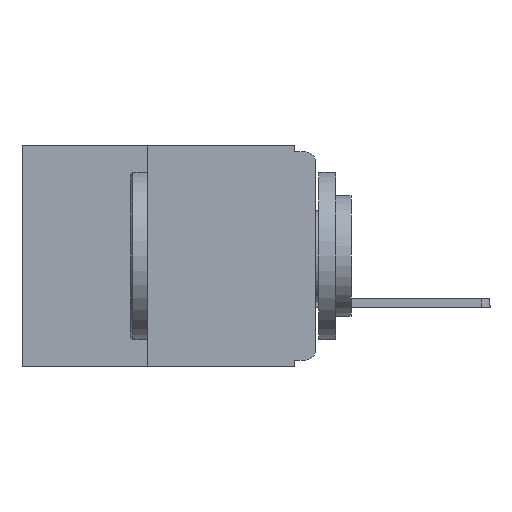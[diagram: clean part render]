
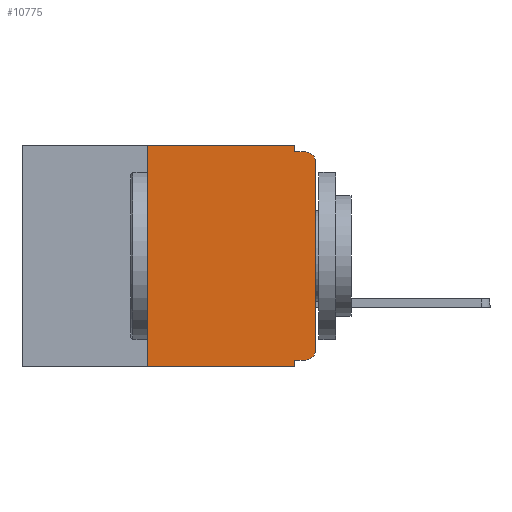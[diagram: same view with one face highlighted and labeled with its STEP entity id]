
A CAD part, left-side view. The second image highlights one B-rep face of the part: STEP entity #10775.
In plain terms, the highlighted planar face has unit normal (-1, 0, 0).
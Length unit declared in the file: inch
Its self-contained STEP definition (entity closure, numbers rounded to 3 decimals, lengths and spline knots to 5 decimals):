
#766 = ORIENTED_EDGE ( 'NONE', *, *, #19208, .F. ) ;
#1764 = DIRECTION ( 'NONE',  ( 0., -1., 0. ) ) ;
#1900 = CARTESIAN_POINT ( 'NONE',  ( 0., 0.015, -0.305 ) ) ;
#2161 = CARTESIAN_POINT ( 'NONE',  ( 0., 0., -0.32 ) ) ;
#3280 = EDGE_LOOP ( 'NONE', ( #29808, #20741, #8644, #12980, #18042, #766, #25653, #30674, #28426, #8640 ) ) ;
#3345 = CARTESIAN_POINT ( 'NONE',  ( 0., 0.25, 0. ) ) ;
#3625 = AXIS2_PLACEMENT_3D ( 'NONE', #1900, #20835, #4644 ) ;
#4491 = LINE ( 'NONE', #29049, #32225 ) ;
#4515 = LINE ( 'NONE', #10232, #24343 ) ;
#4644 = DIRECTION ( 'NONE',  ( 0., 0., -1. ) ) ;
#4915 = DIRECTION ( 'NONE',  ( 0., 1., 0. ) ) ;
#5037 = EDGE_CURVE ( 'NONE', #18623, #21299, #11745, .T. ) ;
#6126 = VECTOR ( 'NONE', #12743, 39.37008 ) ;
#6256 = CARTESIAN_POINT ( 'NONE',  ( 0., 0., -0.305 ) ) ;
#6381 = EDGE_CURVE ( 'NONE', #29842, #32812, #9948, .T. ) ;
#6415 = DIRECTION ( 'NONE',  ( 0., 0., 1. ) ) ;
#6473 = CARTESIAN_POINT ( 'NONE',  ( 0., 0.031, 0. ) ) ;
#6485 = EDGE_CURVE ( 'NONE', #15979, #17301, #20900, .T. ) ;
#7146 = CARTESIAN_POINT ( 'NONE',  ( 0., 0.25, -0.33 ) ) ;
#7497 = DIRECTION ( 'NONE',  ( 0., -1., 0. ) ) ;
#7969 = CARTESIAN_POINT ( 'NONE',  ( 0., 0.015, -0.025 ) ) ;
#8640 = ORIENTED_EDGE ( 'NONE', *, *, #31107, .T. ) ;
#8644 = ORIENTED_EDGE ( 'NONE', *, *, #5037, .F. ) ;
#8775 = CARTESIAN_POINT ( 'NONE',  ( 0., 0., -0.025 ) ) ;
#9948 = LINE ( 'NONE', #2161, #23394 ) ;
#10037 = CARTESIAN_POINT ( 'NONE',  ( 0., 0.031, -0.33 ) ) ;
#10232 = CARTESIAN_POINT ( 'NONE',  ( 0., 0.437, 0. ) ) ;
#10708 = DIRECTION ( 'NONE',  ( 0., 0., -1. ) ) ;
#10775 = ADVANCED_FACE ( 'NONE', ( #24810 ), #29606, .F. ) ;
#11642 = EDGE_CURVE ( 'NONE', #32002, #33208, #32650, .T. ) ;
#11745 = LINE ( 'NONE', #18168, #18114 ) ;
#12477 = CARTESIAN_POINT ( 'NONE',  ( 0., 0.031, -0.32 ) ) ;
#12743 = DIRECTION ( 'NONE',  ( 0., 0., -1. ) ) ;
#12980 = ORIENTED_EDGE ( 'NONE', *, *, #33434, .F. ) ;
#13438 = CARTESIAN_POINT ( 'NONE',  ( 0., 0.437, -0.33 ) ) ;
#13593 = DIRECTION ( 'NONE',  ( 1., 0., 0. ) ) ;
#14656 = LINE ( 'NONE', #20573, #28015 ) ;
#14970 = VERTEX_POINT ( 'NONE', #6473 ) ;
#15979 = VERTEX_POINT ( 'NONE', #7146 ) ;
#16168 = EDGE_CURVE ( 'NONE', #33208, #21299, #20493, .T. ) ;
#16734 = AXIS2_PLACEMENT_3D ( 'NONE', #21576, #13593, #32283 ) ;
#17301 = VERTEX_POINT ( 'NONE', #32049 ) ;
#17327 = CARTESIAN_POINT ( 'NONE',  ( 0., 0., 0. ) ) ;
#17913 = CARTESIAN_POINT ( 'NONE',  ( 0., 0.015, -0.32 ) ) ;
#18042 = ORIENTED_EDGE ( 'NONE', *, *, #32919, .F. ) ;
#18114 = VECTOR ( 'NONE', #1764, 39.37008 ) ;
#18168 = CARTESIAN_POINT ( 'NONE',  ( 0., 0., -0.01 ) ) ;
#18623 = VERTEX_POINT ( 'NONE', #28847 ) ;
#19208 = EDGE_CURVE ( 'NONE', #15979, #30822, #4491, .T. ) ;
#19487 = CARTESIAN_POINT ( 'NONE',  ( 0., 0.015, -0.01 ) ) ;
#20493 = CIRCLE ( 'NONE', #20854, 0.015 ) ;
#20496 = LINE ( 'NONE', #10037, #6126 ) ;
#20573 = CARTESIAN_POINT ( 'NONE',  ( 0., 0.031, 0. ) ) ;
#20741 = ORIENTED_EDGE ( 'NONE', *, *, #16168, .T. ) ;
#20835 = DIRECTION ( 'NONE',  ( -1., 0., 0. ) ) ;
#20854 = AXIS2_PLACEMENT_3D ( 'NONE', #7969, #26765, #10708 ) ;
#20900 = LINE ( 'NONE', #13438, #34212 ) ;
#21138 = DIRECTION ( 'NONE',  ( 0., 0., 1. ) ) ;
#21299 = VERTEX_POINT ( 'NONE', #19487 ) ;
#21576 = CARTESIAN_POINT ( 'NONE',  ( 0., 0.437, 0. ) ) ;
#23394 = VECTOR ( 'NONE', #4915, 39.37008 ) ;
#24343 = VECTOR ( 'NONE', #7497, 39.37008 ) ;
#24810 = FACE_OUTER_BOUND ( 'NONE', #3280, .T. ) ;
#25653 = ORIENTED_EDGE ( 'NONE', *, *, #6485, .T. ) ;
#25939 = DIRECTION ( 'NONE',  ( 0., 0., -1. ) ) ;
#26765 = DIRECTION ( 'NONE',  ( -1., 0., 0. ) ) ;
#26781 = DIRECTION ( 'NONE',  ( 0., -1., 0. ) ) ;
#28015 = VECTOR ( 'NONE', #25939, 39.37008 ) ;
#28426 = ORIENTED_EDGE ( 'NONE', *, *, #6381, .F. ) ;
#28847 = CARTESIAN_POINT ( 'NONE',  ( 0., 0.031, -0.01 ) ) ;
#29049 = CARTESIAN_POINT ( 'NONE',  ( 0., 0.25, -0.33 ) ) ;
#29606 = PLANE ( 'NONE',  #16734 ) ;
#29808 = ORIENTED_EDGE ( 'NONE', *, *, #11642, .T. ) ;
#29842 = VERTEX_POINT ( 'NONE', #17913 ) ;
#30674 = ORIENTED_EDGE ( 'NONE', *, *, #34104, .F. ) ;
#30822 = VERTEX_POINT ( 'NONE', #3345 ) ;
#31107 = EDGE_CURVE ( 'NONE', #29842, #32002, #34423, .T. ) ;
#31824 = VECTOR ( 'NONE', #6415, 39.37008 ) ;
#32002 = VERTEX_POINT ( 'NONE', #6256 ) ;
#32049 = CARTESIAN_POINT ( 'NONE',  ( 0., 0.031, -0.33 ) ) ;
#32225 = VECTOR ( 'NONE', #21138, 39.37008 ) ;
#32283 = DIRECTION ( 'NONE',  ( 0., 0., -1. ) ) ;
#32650 = LINE ( 'NONE', #17327, #31824 ) ;
#32812 = VERTEX_POINT ( 'NONE', #12477 ) ;
#32919 = EDGE_CURVE ( 'NONE', #30822, #14970, #4515, .T. ) ;
#33208 = VERTEX_POINT ( 'NONE', #8775 ) ;
#33434 = EDGE_CURVE ( 'NONE', #14970, #18623, #14656, .T. ) ;
#34104 = EDGE_CURVE ( 'NONE', #32812, #17301, #20496, .T. ) ;
#34212 = VECTOR ( 'NONE', #26781, 39.37008 ) ;
#34423 = CIRCLE ( 'NONE', #3625, 0.015 ) ;
